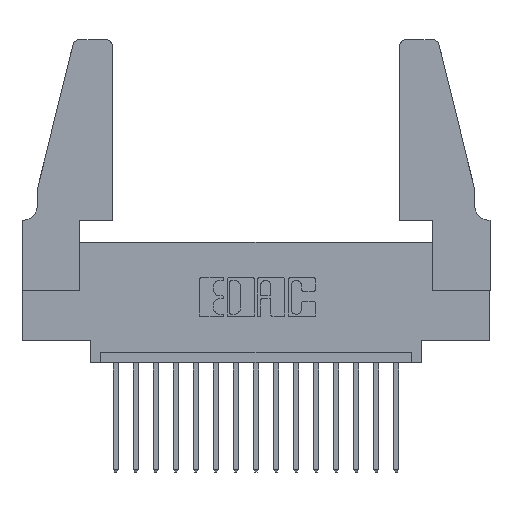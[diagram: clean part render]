
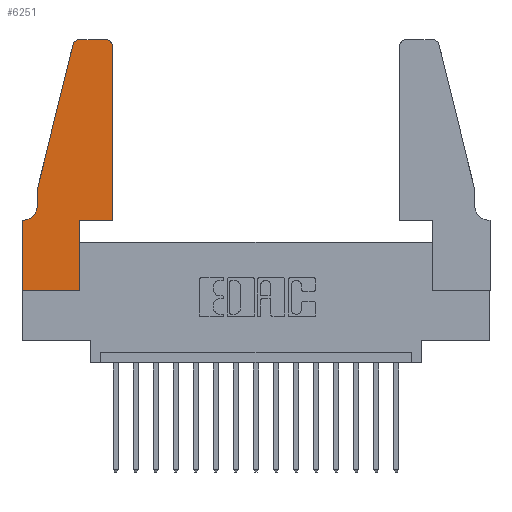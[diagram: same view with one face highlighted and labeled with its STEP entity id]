
A CAD part, top view. The second image highlights one B-rep face of the part: STEP entity #6251.
In plain terms, the highlighted planar face has unit normal (0, 0, 1).
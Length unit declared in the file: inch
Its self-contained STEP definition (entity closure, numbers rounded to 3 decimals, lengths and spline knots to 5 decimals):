
#19 = CARTESIAN_POINT ( 'NONE',  ( 0.0755, 0.5, 0.37 ) ) ;
#220 = ORIENTED_EDGE ( 'NONE', *, *, #9424, .T. ) ;
#393 = CIRCLE ( 'NONE', #9513, 0.07 ) ;
#626 = CARTESIAN_POINT ( 'NONE',  ( 0., 0., 0.37 ) ) ;
#633 = CARTESIAN_POINT ( 'NONE',  ( 0.2865, 0.35, 0.37 ) ) ;
#659 = ORIENTED_EDGE ( 'NONE', *, *, #2870, .T. ) ;
#721 = ORIENTED_EDGE ( 'NONE', *, *, #13102, .T. ) ;
#786 = CARTESIAN_POINT ( 'NONE',  ( 0.284, 1.22, 0.37 ) ) ;
#843 = LINE ( 'NONE', #4216, #8028 ) ;
#1093 = DIRECTION ( 'NONE',  ( 1., 0., 0. ) ) ;
#1254 = CARTESIAN_POINT ( 'NONE',  ( 0.4205, 1.25, 0.37 ) ) ;
#1457 = CARTESIAN_POINT ( 'NONE',  ( 0.25487, 1.22718, 0.37 ) ) ;
#1864 = VERTEX_POINT ( 'NONE', #8621 ) ;
#2212 = DIRECTION ( 'NONE',  ( 0., 1., 0. ) ) ;
#2535 = AXIS2_PLACEMENT_3D ( 'NONE', #786, #7763, #13350 ) ;
#2617 = DIRECTION ( 'NONE',  ( -1., 0., 0. ) ) ;
#2660 = VERTEX_POINT ( 'NONE', #16239 ) ;
#2692 = CARTESIAN_POINT ( 'NONE',  ( 0., 0.35, 0.37 ) ) ;
#2870 = EDGE_CURVE ( 'NONE', #7263, #3038, #16654, .T. ) ;
#2948 = ORIENTED_EDGE ( 'NONE', *, *, #7365, .T. ) ;
#3001 = VERTEX_POINT ( 'NONE', #1457 ) ;
#3038 = VERTEX_POINT ( 'NONE', #12300 ) ;
#3227 = EDGE_CURVE ( 'NONE', #13056, #5846, #15602, .T. ) ;
#3333 = VERTEX_POINT ( 'NONE', #6702 ) ;
#3799 = CARTESIAN_POINT ( 'NONE',  ( 0.4505, 0.35, 0.37 ) ) ;
#4043 = ORIENTED_EDGE ( 'NONE', *, *, #9671, .T. ) ;
#4216 = CARTESIAN_POINT ( 'NONE',  ( 0.4505, 0.35, 0.37 ) ) ;
#4241 = CARTESIAN_POINT ( 'NONE',  ( 0.4505, 0.35, 0.37 ) ) ;
#4407 = DIRECTION ( 'NONE',  ( -1., 0., 0. ) ) ;
#4677 = DIRECTION ( 'NONE',  ( 1., 0., 0. ) ) ;
#4767 = CARTESIAN_POINT ( 'NONE',  ( 0.2865, 0.35, 0.37 ) ) ;
#4810 = VECTOR ( 'NONE', #2212, 39.37008 ) ;
#4969 = ORIENTED_EDGE ( 'NONE', *, *, #10623, .T. ) ;
#5079 = VECTOR ( 'NONE', #4677, 39.37008 ) ;
#5628 = LINE ( 'NONE', #4767, #4810 ) ;
#5846 = VERTEX_POINT ( 'NONE', #15778 ) ;
#6198 = DIRECTION ( 'NONE',  ( 1., 0., 0. ) ) ;
#6251 = ADVANCED_FACE ( 'NONE', ( #10508 ), #15316, .T. ) ;
#6702 = CARTESIAN_POINT ( 'NONE',  ( 0., 0., 0.37 ) ) ;
#6720 = CARTESIAN_POINT ( 'NONE',  ( 0.4505, 1.22, 0.37 ) ) ;
#6805 = CARTESIAN_POINT ( 'NONE',  ( 0.2605, 1.25, 0.37 ) ) ;
#7137 = AXIS2_PLACEMENT_3D ( 'NONE', #2692, #13160, #1093 ) ;
#7263 = VERTEX_POINT ( 'NONE', #13311 ) ;
#7365 = EDGE_CURVE ( 'NONE', #13015, #7621, #13989, .T. ) ;
#7621 = VERTEX_POINT ( 'NONE', #6720 ) ;
#7763 = DIRECTION ( 'NONE',  ( 0., 0., 1. ) ) ;
#7902 = AXIS2_PLACEMENT_3D ( 'NONE', #12788, #12621, #6198 ) ;
#8025 = VECTOR ( 'NONE', #14404, 39.37008 ) ;
#8028 = VECTOR ( 'NONE', #10898, 39.37008 ) ;
#8063 = ORIENTED_EDGE ( 'NONE', *, *, #8275, .T. ) ;
#8275 = EDGE_CURVE ( 'NONE', #5846, #3001, #16080, .T. ) ;
#8510 = DIRECTION ( 'NONE',  ( 0., 0., -1. ) ) ;
#8621 = CARTESIAN_POINT ( 'NONE',  ( 0.2865, 0., 0.37 ) ) ;
#8623 = LINE ( 'NONE', #626, #5079 ) ;
#8884 = EDGE_CURVE ( 'NONE', #3038, #2660, #393, .T. ) ;
#9088 = ORIENTED_EDGE ( 'NONE', *, *, #8884, .T. ) ;
#9151 = VERTEX_POINT ( 'NONE', #633 ) ;
#9276 = DIRECTION ( 'NONE',  ( 0., -1., 0. ) ) ;
#9350 = VECTOR ( 'NONE', #17030, 39.37008 ) ;
#9424 = EDGE_CURVE ( 'NONE', #3333, #1864, #8623, .T. ) ;
#9513 = AXIS2_PLACEMENT_3D ( 'NONE', #11089, #8510, #12231 ) ;
#9671 = EDGE_CURVE ( 'NONE', #3001, #7263, #10874, .T. ) ;
#10324 = VECTOR ( 'NONE', #4407, 39.37008 ) ;
#10425 = VECTOR ( 'NONE', #2617, 39.37008 ) ;
#10508 = FACE_OUTER_BOUND ( 'NONE', #14241, .T. ) ;
#10528 = LINE ( 'NONE', #14097, #10324 ) ;
#10623 = EDGE_CURVE ( 'NONE', #1864, #9151, #5628, .T. ) ;
#10874 = LINE ( 'NONE', #13286, #11073 ) ;
#10898 = DIRECTION ( 'NONE',  ( 1., 0., 0. ) ) ;
#11073 = VECTOR ( 'NONE', #12293, 39.37008 ) ;
#11089 = CARTESIAN_POINT ( 'NONE',  ( 0.0055, 0.42, 0.37 ) ) ;
#12147 = ORIENTED_EDGE ( 'NONE', *, *, #3227, .T. ) ;
#12215 = ORIENTED_EDGE ( 'NONE', *, *, #15148, .T. ) ;
#12231 = DIRECTION ( 'NONE',  ( -1., 0., 0. ) ) ;
#12293 = DIRECTION ( 'NONE',  ( -0.239, -0.971, 0. ) ) ;
#12300 = CARTESIAN_POINT ( 'NONE',  ( 0.0755, 0.42, 0.37 ) ) ;
#12621 = DIRECTION ( 'NONE',  ( 0., 0., 1. ) ) ;
#12788 = CARTESIAN_POINT ( 'NONE',  ( 0.4205, 1.22, 0.37 ) ) ;
#13015 = VERTEX_POINT ( 'NONE', #4241 ) ;
#13056 = VERTEX_POINT ( 'NONE', #1254 ) ;
#13102 = EDGE_CURVE ( 'NONE', #2660, #15511, #10528, .T. ) ;
#13160 = DIRECTION ( 'NONE',  ( 0., 0., 1. ) ) ;
#13248 = LINE ( 'NONE', #16981, #9350 ) ;
#13286 = CARTESIAN_POINT ( 'NONE',  ( 0.0755, 0.5, 0.37 ) ) ;
#13311 = CARTESIAN_POINT ( 'NONE',  ( 0.0755, 0.5, 0.37 ) ) ;
#13350 = DIRECTION ( 'NONE',  ( 1., 0., 0. ) ) ;
#13364 = ORIENTED_EDGE ( 'NONE', *, *, #13794, .T. ) ;
#13757 = CARTESIAN_POINT ( 'NONE',  ( 0., 0.35, 0.37 ) ) ;
#13794 = EDGE_CURVE ( 'NONE', #9151, #13015, #843, .T. ) ;
#13989 = LINE ( 'NONE', #3799, #8025 ) ;
#14097 = CARTESIAN_POINT ( 'NONE',  ( 0.0755, 0.35, 0.37 ) ) ;
#14241 = EDGE_LOOP ( 'NONE', ( #12147, #8063, #4043, #659, #9088, #721, #12215, #220, #4969, #13364, #2948, #16817 ) ) ;
#14404 = DIRECTION ( 'NONE',  ( 0., 1., 0. ) ) ;
#14781 = VECTOR ( 'NONE', #9276, 39.37008 ) ;
#14881 = EDGE_CURVE ( 'NONE', #7621, #13056, #15762, .T. ) ;
#15148 = EDGE_CURVE ( 'NONE', #15511, #3333, #13248, .T. ) ;
#15316 = PLANE ( 'NONE',  #7137 ) ;
#15511 = VERTEX_POINT ( 'NONE', #13757 ) ;
#15602 = LINE ( 'NONE', #6805, #10425 ) ;
#15762 = CIRCLE ( 'NONE', #7902, 0.03 ) ;
#15778 = CARTESIAN_POINT ( 'NONE',  ( 0.284, 1.25, 0.37 ) ) ;
#16080 = CIRCLE ( 'NONE', #2535, 0.03 ) ;
#16239 = CARTESIAN_POINT ( 'NONE',  ( 0.0055, 0.35, 0.37 ) ) ;
#16654 = LINE ( 'NONE', #19, #14781 ) ;
#16817 = ORIENTED_EDGE ( 'NONE', *, *, #14881, .T. ) ;
#16981 = CARTESIAN_POINT ( 'NONE',  ( 0., 0., 0.37 ) ) ;
#17030 = DIRECTION ( 'NONE',  ( 0., -1., 0. ) ) ;
